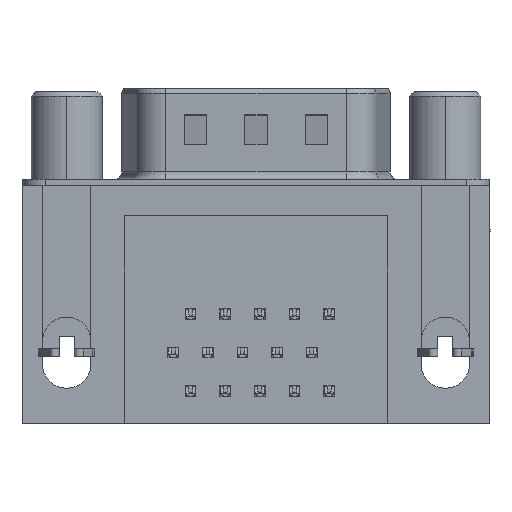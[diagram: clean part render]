
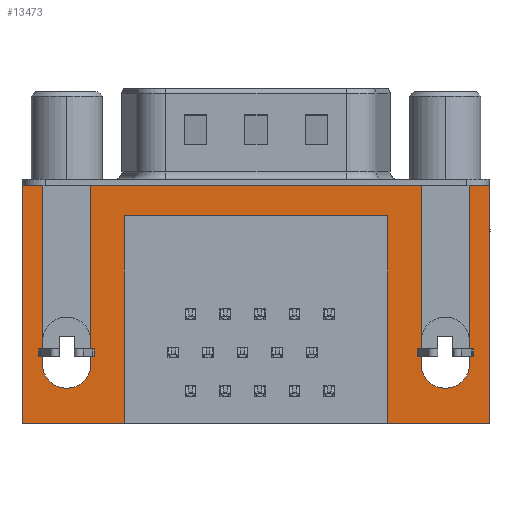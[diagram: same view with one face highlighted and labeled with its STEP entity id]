
A CAD part, front view. The second image highlights one B-rep face of the part: STEP entity #13473.
In plain terms, the highlighted planar face has unit normal (0, -1, 0).
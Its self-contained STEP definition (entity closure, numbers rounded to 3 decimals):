
#369 = DIRECTION ( 'NONE',  ( 0., 0., 1. ) ) ;
#587 = VECTOR ( 'NONE', #20222, 1000. ) ;
#815 = ORIENTED_EDGE ( 'NONE', *, *, #13650, .F. ) ;
#861 = CARTESIAN_POINT ( 'NONE',  ( 26.59, -6.275, -11.78 ) ) ;
#875 = EDGE_CURVE ( 'NONE', #20285, #6772, #6167, .T. ) ;
#928 = CIRCLE ( 'NONE', #17999, 1.6 ) ;
#1168 = LINE ( 'NONE', #6915, #19315 ) ;
#1208 = EDGE_CURVE ( 'NONE', #11263, #15557, #12999, .T. ) ;
#1309 = CARTESIAN_POINT ( 'NONE',  ( 21.2, -6.275, -2. ) ) ;
#1398 = ORIENTED_EDGE ( 'NONE', *, *, #875, .F. ) ;
#1602 = CARTESIAN_POINT ( 'NONE',  ( -2.91, -6.275, 0. ) ) ;
#1677 = EDGE_LOOP ( 'NONE', ( #1398, #20221, #4333, #18237, #21677, #3254, #13579, #16274, #4330, #3006, #21815, #12156, #19549, #12080, #11978, #6544, #1997, #815 ) ) ;
#1837 = CARTESIAN_POINT ( 'NONE',  ( 0., -6.275, -13.38 ) ) ;
#1855 = PLANE ( 'NONE',  #19585 ) ;
#1997 = ORIENTED_EDGE ( 'NONE', *, *, #19425, .T. ) ;
#2066 = EDGE_CURVE ( 'NONE', #20566, #17452, #1168, .T. ) ;
#2264 = CARTESIAN_POINT ( 'NONE',  ( -2.91, -6.275, 0. ) ) ;
#3006 = ORIENTED_EDGE ( 'NONE', *, *, #14351, .F. ) ;
#3034 = EDGE_CURVE ( 'NONE', #20479, #9061, #21463, .T. ) ;
#3254 = ORIENTED_EDGE ( 'NONE', *, *, #1208, .F. ) ;
#3282 = VERTEX_POINT ( 'NONE', #13567 ) ;
#3312 = CARTESIAN_POINT ( 'NONE',  ( 3.79, -6.275, -15.7 ) ) ;
#3382 = DIRECTION ( 'NONE',  ( 0., 0., 1. ) ) ;
#3507 = DIRECTION ( 'NONE',  ( 0., 0., -1. ) ) ;
#3509 = EDGE_CURVE ( 'NONE', #22004, #20285, #9090, .T. ) ;
#3534 = CARTESIAN_POINT ( 'NONE',  ( 0., -6.275, -11.78 ) ) ;
#3734 = CARTESIAN_POINT ( 'NONE',  ( 24.99, -6.275, -11.78 ) ) ;
#3766 = DIRECTION ( 'NONE',  ( 0., -1., 0. ) ) ;
#3772 = AXIS2_PLACEMENT_3D ( 'NONE', #4832, #17135, #6591 ) ;
#3953 = DIRECTION ( 'NONE',  ( 1., 0., 0. ) ) ;
#4330 = ORIENTED_EDGE ( 'NONE', *, *, #17549, .F. ) ;
#4333 = ORIENTED_EDGE ( 'NONE', *, *, #9506, .F. ) ;
#4468 = CARTESIAN_POINT ( 'NONE',  ( 3.79, -6.275, -2. ) ) ;
#4613 = CARTESIAN_POINT ( 'NONE',  ( -1.6, -6.275, 0. ) ) ;
#4797 = CARTESIAN_POINT ( 'NONE',  ( 26.59, -6.275, 0. ) ) ;
#4832 = CARTESIAN_POINT ( 'NONE',  ( 24.99, -6.275, -11.78 ) ) ;
#4892 = CARTESIAN_POINT ( 'NONE',  ( 26.59, -6.275, 0. ) ) ;
#5144 = CARTESIAN_POINT ( 'NONE',  ( 3.79, -6.275, -2. ) ) ;
#5250 = LINE ( 'NONE', #6161, #587 ) ;
#5268 = DIRECTION ( 'NONE',  ( 0., 0., -1. ) ) ;
#5307 = DIRECTION ( 'NONE',  ( 0., 0., -1. ) ) ;
#5426 = EDGE_CURVE ( 'NONE', #10901, #20566, #17305, .T. ) ;
#5455 = DIRECTION ( 'NONE',  ( 0., 0., 1. ) ) ;
#5706 = LINE ( 'NONE', #2264, #18625 ) ;
#5921 = CARTESIAN_POINT ( 'NONE',  ( -2.91, -6.275, 0. ) ) ;
#6161 = CARTESIAN_POINT ( 'NONE',  ( 27.9, -6.275, -15.7 ) ) ;
#6167 = LINE ( 'NONE', #4797, #14963 ) ;
#6236 = CARTESIAN_POINT ( 'NONE',  ( 23.39, -6.275, 0. ) ) ;
#6270 = VERTEX_POINT ( 'NONE', #10493 ) ;
#6366 = CARTESIAN_POINT ( 'NONE',  ( 21.2, -6.275, -2. ) ) ;
#6544 = ORIENTED_EDGE ( 'NONE', *, *, #13071, .F. ) ;
#6591 = DIRECTION ( 'NONE',  ( 0., 0., 1. ) ) ;
#6693 = LINE ( 'NONE', #5921, #11333 ) ;
#6772 = VERTEX_POINT ( 'NONE', #4892 ) ;
#6915 = CARTESIAN_POINT ( 'NONE',  ( 27.9, -6.275, -15.7 ) ) ;
#7079 = CARTESIAN_POINT ( 'NONE',  ( 1.6, -6.275, -11.78 ) ) ;
#7100 = CARTESIAN_POINT ( 'NONE',  ( 27.9, -6.275, -15.7 ) ) ;
#7206 = EDGE_CURVE ( 'NONE', #17452, #14026, #16736, .T. ) ;
#7381 = VECTOR ( 'NONE', #8095, 1000. ) ;
#7936 = CARTESIAN_POINT ( 'NONE',  ( 3.79, -6.275, -2. ) ) ;
#8037 = CARTESIAN_POINT ( 'NONE',  ( -2.91, -6.275, 0. ) ) ;
#8038 = VECTOR ( 'NONE', #15674, 1000. ) ;
#8095 = DIRECTION ( 'NONE',  ( 0., 0., 1. ) ) ;
#8904 = VECTOR ( 'NONE', #9496, 1000. ) ;
#8918 = DIRECTION ( 'NONE',  ( 0., -1., 0. ) ) ;
#9000 = EDGE_CURVE ( 'NONE', #3282, #16673, #13312, .T. ) ;
#9061 = VERTEX_POINT ( 'NONE', #20810 ) ;
#9090 = CIRCLE ( 'NONE', #17477, 1.6 ) ;
#9496 = DIRECTION ( 'NONE',  ( 0., 0., 1. ) ) ;
#9506 = EDGE_CURVE ( 'NONE', #9061, #22004, #18032, .T. ) ;
#9579 = CARTESIAN_POINT ( 'NONE',  ( 0., -6.275, -11.78 ) ) ;
#10118 = CARTESIAN_POINT ( 'NONE',  ( 23.39, -6.275, 0. ) ) ;
#10237 = CARTESIAN_POINT ( 'NONE',  ( -2.91, -6.275, -15.7 ) ) ;
#10461 = CARTESIAN_POINT ( 'NONE',  ( -1.6, -6.275, 0. ) ) ;
#10493 = CARTESIAN_POINT ( 'NONE',  ( -1.6, -6.275, -11.78 ) ) ;
#10866 = CARTESIAN_POINT ( 'NONE',  ( 27.9, -6.275, -2.5 ) ) ;
#10901 = VERTEX_POINT ( 'NONE', #7936 ) ;
#11113 = DIRECTION ( 'NONE',  ( -1., 0., 0. ) ) ;
#11263 = VERTEX_POINT ( 'NONE', #7079 ) ;
#11333 = VECTOR ( 'NONE', #18230, 1000. ) ;
#11336 = DIRECTION ( 'NONE',  ( 0., 0., -1. ) ) ;
#11486 = VECTOR ( 'NONE', #18890, 1000. ) ;
#11804 = EDGE_CURVE ( 'NONE', #16673, #10901, #12682, .T. ) ;
#11978 = ORIENTED_EDGE ( 'NONE', *, *, #9000, .F. ) ;
#12080 = ORIENTED_EDGE ( 'NONE', *, *, #11804, .F. ) ;
#12156 = ORIENTED_EDGE ( 'NONE', *, *, #2066, .F. ) ;
#12337 = CARTESIAN_POINT ( 'NONE',  ( -2.91, -6.275, -2.5 ) ) ;
#12504 = VECTOR ( 'NONE', #369, 1000. ) ;
#12682 = LINE ( 'NONE', #5144, #8038 ) ;
#12999 = LINE ( 'NONE', #18359, #8904 ) ;
#13071 = EDGE_CURVE ( 'NONE', #21499, #3282, #5250, .T. ) ;
#13312 = LINE ( 'NONE', #1309, #17492 ) ;
#13473 = ADVANCED_FACE ( 'NONE', ( #15222 ), #1855, .T. ) ;
#13567 = CARTESIAN_POINT ( 'NONE',  ( 21.2, -6.275, -15.7 ) ) ;
#13579 = ORIENTED_EDGE ( 'NONE', *, *, #13731, .F. ) ;
#13650 = EDGE_CURVE ( 'NONE', #6772, #15976, #6693, .T. ) ;
#13731 = EDGE_CURVE ( 'NONE', #20651, #11263, #928, .T. ) ;
#14026 = VERTEX_POINT ( 'NONE', #1602 ) ;
#14351 = EDGE_CURVE ( 'NONE', #14026, #20391, #22565, .T. ) ;
#14535 = CIRCLE ( 'NONE', #17932, 1.6 ) ;
#14963 = VECTOR ( 'NONE', #5455, 1000. ) ;
#15085 = CARTESIAN_POINT ( 'NONE',  ( -2.91, -6.275, -2.5 ) ) ;
#15222 = FACE_OUTER_BOUND ( 'NONE', #1677, .T. ) ;
#15375 = DIRECTION ( 'NONE',  ( 0., 0., 1. ) ) ;
#15557 = VERTEX_POINT ( 'NONE', #18235 ) ;
#15674 = DIRECTION ( 'NONE',  ( -1., 0., 0. ) ) ;
#15828 = DIRECTION ( 'NONE',  ( 0., -1., 0. ) ) ;
#15976 = VERTEX_POINT ( 'NONE', #17807 ) ;
#16274 = ORIENTED_EDGE ( 'NONE', *, *, #20618, .F. ) ;
#16485 = VECTOR ( 'NONE', #5268, 1000. ) ;
#16673 = VERTEX_POINT ( 'NONE', #6366 ) ;
#16736 = LINE ( 'NONE', #15085, #7381 ) ;
#17135 = DIRECTION ( 'NONE',  ( 0., -1., 0. ) ) ;
#17305 = LINE ( 'NONE', #4468, #11486 ) ;
#17452 = VERTEX_POINT ( 'NONE', #10237 ) ;
#17477 = AXIS2_PLACEMENT_3D ( 'NONE', #3734, #3766, #3382 ) ;
#17492 = VECTOR ( 'NONE', #15375, 1000. ) ;
#17549 = EDGE_CURVE ( 'NONE', #20391, #6270, #21111, .T. ) ;
#17807 = CARTESIAN_POINT ( 'NONE',  ( 27.9, -6.275, 0. ) ) ;
#17931 = CARTESIAN_POINT ( 'NONE',  ( 24.99, -6.275, -13.38 ) ) ;
#17932 = AXIS2_PLACEMENT_3D ( 'NONE', #3534, #15828, #5307 ) ;
#17968 = VECTOR ( 'NONE', #20324, 1000. ) ;
#17999 = AXIS2_PLACEMENT_3D ( 'NONE', #9579, #21862, #11336 ) ;
#18032 = CIRCLE ( 'NONE', #3772, 1.6 ) ;
#18230 = DIRECTION ( 'NONE',  ( 1., 0., 0. ) ) ;
#18235 = CARTESIAN_POINT ( 'NONE',  ( 1.6, -6.275, 0. ) ) ;
#18237 = ORIENTED_EDGE ( 'NONE', *, *, #3034, .F. ) ;
#18359 = CARTESIAN_POINT ( 'NONE',  ( 1.6, -6.275, 0. ) ) ;
#18625 = VECTOR ( 'NONE', #3953, 1000. ) ;
#18890 = DIRECTION ( 'NONE',  ( 0., 0., -1. ) ) ;
#19315 = VECTOR ( 'NONE', #11113, 1000. ) ;
#19425 = EDGE_CURVE ( 'NONE', #21499, #15976, #22411, .T. ) ;
#19549 = ORIENTED_EDGE ( 'NONE', *, *, #5426, .F. ) ;
#19585 = AXIS2_PLACEMENT_3D ( 'NONE', #12337, #8918, #21191 ) ;
#20221 = ORIENTED_EDGE ( 'NONE', *, *, #3509, .F. ) ;
#20222 = DIRECTION ( 'NONE',  ( -1., 0., 0. ) ) ;
#20285 = VERTEX_POINT ( 'NONE', #861 ) ;
#20324 = DIRECTION ( 'NONE',  ( 1., 0., 0. ) ) ;
#20367 = VECTOR ( 'NONE', #3507, 1000. ) ;
#20391 = VERTEX_POINT ( 'NONE', #4613 ) ;
#20479 = VERTEX_POINT ( 'NONE', #10118 ) ;
#20566 = VERTEX_POINT ( 'NONE', #3312 ) ;
#20618 = EDGE_CURVE ( 'NONE', #6270, #20651, #14535, .T. ) ;
#20651 = VERTEX_POINT ( 'NONE', #1837 ) ;
#20810 = CARTESIAN_POINT ( 'NONE',  ( 23.39, -6.275, -11.78 ) ) ;
#21111 = LINE ( 'NONE', #10461, #16485 ) ;
#21191 = DIRECTION ( 'NONE',  ( 0., 0., -1. ) ) ;
#21463 = LINE ( 'NONE', #6236, #20367 ) ;
#21499 = VERTEX_POINT ( 'NONE', #7100 ) ;
#21677 = ORIENTED_EDGE ( 'NONE', *, *, #21679, .F. ) ;
#21679 = EDGE_CURVE ( 'NONE', #15557, #20479, #5706, .T. ) ;
#21815 = ORIENTED_EDGE ( 'NONE', *, *, #7206, .F. ) ;
#21862 = DIRECTION ( 'NONE',  ( 0., -1., 0. ) ) ;
#22004 = VERTEX_POINT ( 'NONE', #17931 ) ;
#22411 = LINE ( 'NONE', #10866, #12504 ) ;
#22565 = LINE ( 'NONE', #8037, #17968 ) ;
